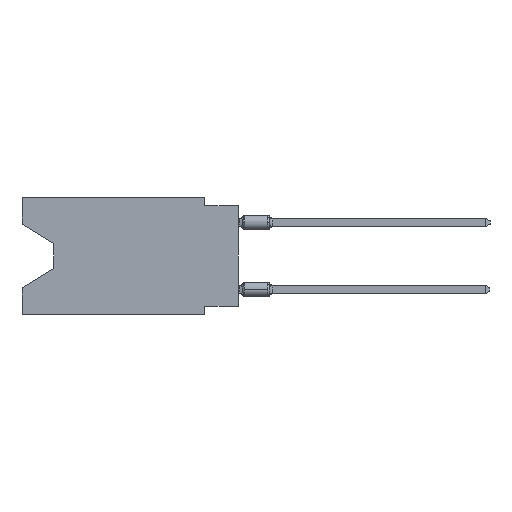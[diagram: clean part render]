
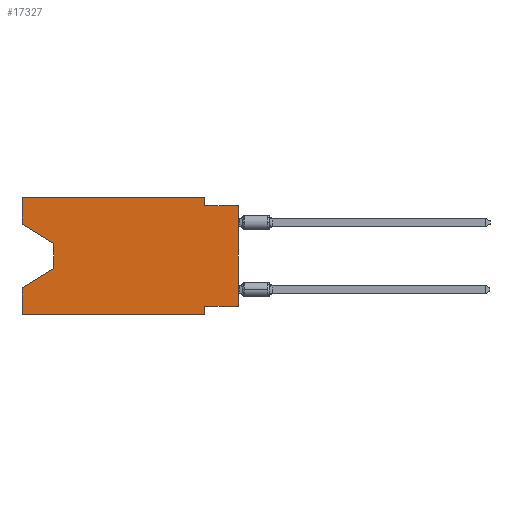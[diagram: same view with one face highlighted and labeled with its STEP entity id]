
A CAD part, left-side view. The second image highlights one B-rep face of the part: STEP entity #17327.
In plain terms, the highlighted planar face has unit normal (-1, 0, 0).
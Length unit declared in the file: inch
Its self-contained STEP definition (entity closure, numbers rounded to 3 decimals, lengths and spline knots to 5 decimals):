
#148 = CARTESIAN_POINT ( 'NONE',  ( 0., 0.55, -0.138 ) ) ;
#275 = FACE_OUTER_BOUND ( 'NONE', #15115, .T. ) ;
#285 = DIRECTION ( 'NONE',  ( 0., 0., -1. ) ) ;
#830 = ORIENTED_EDGE ( 'NONE', *, *, #19898, .F. ) ;
#1951 = CARTESIAN_POINT ( 'NONE',  ( 0., 0.1, -0.025 ) ) ;
#1958 = CARTESIAN_POINT ( 'NONE',  ( 0., 0., -0.325 ) ) ;
#2023 = LINE ( 'NONE', #10494, #19961 ) ;
#2271 = ORIENTED_EDGE ( 'NONE', *, *, #17337, .T. ) ;
#2297 = ORIENTED_EDGE ( 'NONE', *, *, #27360, .T. ) ;
#2371 = CARTESIAN_POINT ( 'NONE',  ( 0., 0.645, 0. ) ) ;
#3221 = EDGE_CURVE ( 'NONE', #22198, #14313, #15763, .T. ) ;
#3268 = CARTESIAN_POINT ( 'NONE',  ( 0., 0., -0.025 ) ) ;
#3900 = ORIENTED_EDGE ( 'NONE', *, *, #18059, .F. ) ;
#4039 = EDGE_CURVE ( 'NONE', #18440, #23087, #20146, .T. ) ;
#4121 = LINE ( 'NONE', #6656, #13017 ) ;
#4132 = DIRECTION ( 'NONE',  ( 0., 0., 1. ) ) ;
#4807 = CARTESIAN_POINT ( 'NONE',  ( 0., 0.645, -0.08025 ) ) ;
#4836 = VERTEX_POINT ( 'NONE', #26024 ) ;
#4938 = CARTESIAN_POINT ( 'NONE',  ( 0., 0.645, -0.26975 ) ) ;
#5163 = VERTEX_POINT ( 'NONE', #25297 ) ;
#5542 = VERTEX_POINT ( 'NONE', #14472 ) ;
#6152 = VECTOR ( 'NONE', #27827, 39.37008 ) ;
#6656 = CARTESIAN_POINT ( 'NONE',  ( 0., 0., -0.325 ) ) ;
#6757 = DIRECTION ( 'NONE',  ( 0., 0., -1. ) ) ;
#6912 = CARTESIAN_POINT ( 'NONE',  ( 0., 0.1, -0.35 ) ) ;
#7123 = DIRECTION ( 'NONE',  ( 0., 0.855, -0.519 ) ) ;
#7132 = AXIS2_PLACEMENT_3D ( 'NONE', #2371, #13122, #15223 ) ;
#7586 = VECTOR ( 'NONE', #18637, 39.37008 ) ;
#7663 = DIRECTION ( 'NONE',  ( 0., 0., 1. ) ) ;
#7918 = LINE ( 'NONE', #25551, #8988 ) ;
#8646 = CARTESIAN_POINT ( 'NONE',  ( 0., 0.1, -0.35 ) ) ;
#8872 = PLANE ( 'NONE',  #7132 ) ;
#8988 = VECTOR ( 'NONE', #14847, 39.37008 ) ;
#9247 = LINE ( 'NONE', #24068, #19162 ) ;
#9622 = LINE ( 'NONE', #3268, #7586 ) ;
#9626 = ORIENTED_EDGE ( 'NONE', *, *, #24623, .T. ) ;
#9993 = CARTESIAN_POINT ( 'NONE',  ( 0., 0.1, -0.325 ) ) ;
#10471 = EDGE_CURVE ( 'NONE', #4836, #23805, #2023, .T. ) ;
#10494 = CARTESIAN_POINT ( 'NONE',  ( 0., 0.645, 0. ) ) ;
#10617 = CARTESIAN_POINT ( 'NONE',  ( 0., 0.645, -0.35 ) ) ;
#10930 = ORIENTED_EDGE ( 'NONE', *, *, #19158, .T. ) ;
#11603 = VERTEX_POINT ( 'NONE', #9993 ) ;
#12176 = ORIENTED_EDGE ( 'NONE', *, *, #4039, .F. ) ;
#12460 = LINE ( 'NONE', #14437, #16129 ) ;
#12836 = VECTOR ( 'NONE', #22249, 39.37008 ) ;
#13017 = VECTOR ( 'NONE', #15269, 39.37008 ) ;
#13122 = DIRECTION ( 'NONE',  ( 1., 0., 0. ) ) ;
#13856 = CARTESIAN_POINT ( 'NONE',  ( 0., 0., 0. ) ) ;
#13966 = VERTEX_POINT ( 'NONE', #1958 ) ;
#14313 = VERTEX_POINT ( 'NONE', #26043 ) ;
#14355 = VECTOR ( 'NONE', #6757, 39.37008 ) ;
#14437 = CARTESIAN_POINT ( 'NONE',  ( 0., 0.645, 0. ) ) ;
#14472 = CARTESIAN_POINT ( 'NONE',  ( 0., 0.645, 0. ) ) ;
#14762 = CARTESIAN_POINT ( 'NONE',  ( 0., 0.1, 0. ) ) ;
#14847 = DIRECTION ( 'NONE',  ( 0., -1., 0. ) ) ;
#15005 = EDGE_CURVE ( 'NONE', #23087, #5163, #9622, .T. ) ;
#15115 = EDGE_LOOP ( 'NONE', ( #19724, #2271, #9626, #26023, #2297, #16230, #830, #10930, #15498, #12176, #3900, #18155 ) ) ;
#15223 = DIRECTION ( 'NONE',  ( 0., 0., -1. ) ) ;
#15269 = DIRECTION ( 'NONE',  ( 0., 1., 0. ) ) ;
#15498 = ORIENTED_EDGE ( 'NONE', *, *, #15005, .F. ) ;
#15763 = LINE ( 'NONE', #22382, #12836 ) ;
#16126 = CARTESIAN_POINT ( 'NONE',  ( 0., 0.55, -0.212 ) ) ;
#16129 = VECTOR ( 'NONE', #7663, 39.37008 ) ;
#16230 = ORIENTED_EDGE ( 'NONE', *, *, #23606, .F. ) ;
#16567 = VECTOR ( 'NONE', #24579, 39.37008 ) ;
#17192 = LINE ( 'NONE', #148, #14355 ) ;
#17272 = VECTOR ( 'NONE', #285, 39.37008 ) ;
#17327 = ADVANCED_FACE ( 'NONE', ( #275 ), #8872, .F. ) ;
#17337 = EDGE_CURVE ( 'NONE', #14313, #19663, #17192, .T. ) ;
#18059 = EDGE_CURVE ( 'NONE', #5542, #18440, #7918, .T. ) ;
#18088 = LINE ( 'NONE', #13856, #16567 ) ;
#18155 = ORIENTED_EDGE ( 'NONE', *, *, #19660, .F. ) ;
#18440 = VERTEX_POINT ( 'NONE', #14762 ) ;
#18637 = DIRECTION ( 'NONE',  ( 0., -1., 0. ) ) ;
#19158 = EDGE_CURVE ( 'NONE', #13966, #5163, #18088, .T. ) ;
#19162 = VECTOR ( 'NONE', #7123, 39.37008 ) ;
#19660 = EDGE_CURVE ( 'NONE', #22198, #5542, #12460, .T. ) ;
#19663 = VERTEX_POINT ( 'NONE', #16126 ) ;
#19724 = ORIENTED_EDGE ( 'NONE', *, *, #3221, .T. ) ;
#19898 = EDGE_CURVE ( 'NONE', #13966, #11603, #4121, .T. ) ;
#19961 = VECTOR ( 'NONE', #4132, 39.37008 ) ;
#20146 = LINE ( 'NONE', #24395, #17272 ) ;
#21342 = LINE ( 'NONE', #10617, #6152 ) ;
#21817 = VECTOR ( 'NONE', #25973, 39.37008 ) ;
#21871 = LINE ( 'NONE', #8646, #21817 ) ;
#22198 = VERTEX_POINT ( 'NONE', #4807 ) ;
#22249 = DIRECTION ( 'NONE',  ( 0., -0.855, -0.519 ) ) ;
#22382 = CARTESIAN_POINT ( 'NONE',  ( 0., 0.645, -0.08025 ) ) ;
#22615 = VERTEX_POINT ( 'NONE', #6912 ) ;
#23087 = VERTEX_POINT ( 'NONE', #1951 ) ;
#23606 = EDGE_CURVE ( 'NONE', #11603, #22615, #21871, .T. ) ;
#23805 = VERTEX_POINT ( 'NONE', #4938 ) ;
#24068 = CARTESIAN_POINT ( 'NONE',  ( 0., 0.55, -0.212 ) ) ;
#24395 = CARTESIAN_POINT ( 'NONE',  ( 0., 0.1, 0. ) ) ;
#24579 = DIRECTION ( 'NONE',  ( 0., 0., 1. ) ) ;
#24623 = EDGE_CURVE ( 'NONE', #19663, #23805, #9247, .T. ) ;
#25297 = CARTESIAN_POINT ( 'NONE',  ( 0., 0., -0.025 ) ) ;
#25551 = CARTESIAN_POINT ( 'NONE',  ( 0., 0.645, 0. ) ) ;
#25973 = DIRECTION ( 'NONE',  ( 0., 0., -1. ) ) ;
#26023 = ORIENTED_EDGE ( 'NONE', *, *, #10471, .F. ) ;
#26024 = CARTESIAN_POINT ( 'NONE',  ( 0., 0.645, -0.35 ) ) ;
#26043 = CARTESIAN_POINT ( 'NONE',  ( 0., 0.55, -0.138 ) ) ;
#27360 = EDGE_CURVE ( 'NONE', #4836, #22615, #21342, .T. ) ;
#27827 = DIRECTION ( 'NONE',  ( 0., -1., 0. ) ) ;
